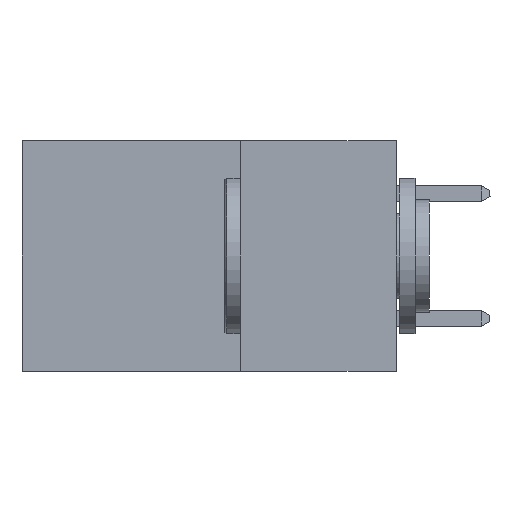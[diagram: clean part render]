
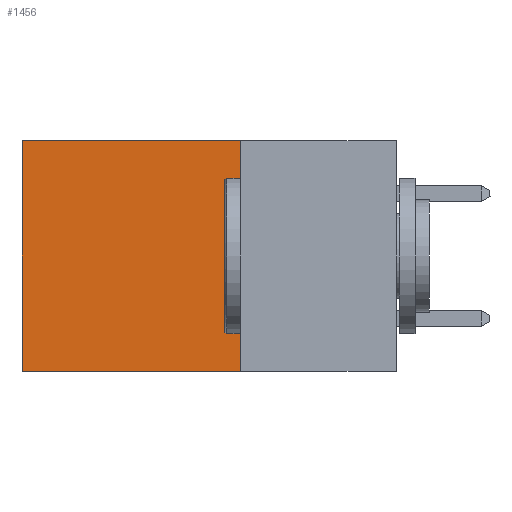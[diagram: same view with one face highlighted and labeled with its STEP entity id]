
A CAD part, left-side view. The second image highlights one B-rep face of the part: STEP entity #1456.
In plain terms, the highlighted planar face has unit normal (-1, 0, 0).
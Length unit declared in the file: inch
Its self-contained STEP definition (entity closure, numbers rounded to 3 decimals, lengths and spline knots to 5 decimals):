
#746 = LINE ( 'NONE', #5062, #2712 ) ;
#984 = VERTEX_POINT ( 'NONE', #23093 ) ;
#1456 = ADVANCED_FACE ( 'NONE', ( #5868 ), #20623, .F. ) ;
#1701 = ORIENTED_EDGE ( 'NONE', *, *, #24674, .T. ) ;
#1760 = VECTOR ( 'NONE', #31688, 39.37008 ) ;
#1788 = DIRECTION ( 'NONE',  ( 0., 1., 0. ) ) ;
#1987 = ORIENTED_EDGE ( 'NONE', *, *, #8417, .F. ) ;
#2712 = VECTOR ( 'NONE', #17250, 39.37008 ) ;
#3353 = LINE ( 'NONE', #26395, #1760 ) ;
#4604 = EDGE_LOOP ( 'NONE', ( #29391, #16786, #1987, #1701 ) ) ;
#5062 = CARTESIAN_POINT ( 'NONE',  ( 0.298, 0.25, -0.37 ) ) ;
#5517 = DIRECTION ( 'NONE',  ( 0., 0., -1. ) ) ;
#5868 = FACE_OUTER_BOUND ( 'NONE', #4604, .T. ) ;
#7280 = EDGE_CURVE ( 'NONE', #13298, #9514, #746, .T. ) ;
#8139 = VERTEX_POINT ( 'NONE', #17391 ) ;
#8417 = EDGE_CURVE ( 'NONE', #8139, #13298, #14065, .T. ) ;
#9514 = VERTEX_POINT ( 'NONE', #31821 ) ;
#9666 = DIRECTION ( 'NONE',  ( 0., 0., -1. ) ) ;
#13298 = VERTEX_POINT ( 'NONE', #14945 ) ;
#14065 = LINE ( 'NONE', #29953, #25134 ) ;
#14945 = CARTESIAN_POINT ( 'NONE',  ( 0.298, 0.25, -0.37 ) ) ;
#15880 = LINE ( 'NONE', #29448, #20218 ) ;
#16786 = ORIENTED_EDGE ( 'NONE', *, *, #7280, .F. ) ;
#17250 = DIRECTION ( 'NONE',  ( 0., 1., 0. ) ) ;
#17391 = CARTESIAN_POINT ( 'NONE',  ( 0.298, 0.25, 0. ) ) ;
#18501 = AXIS2_PLACEMENT_3D ( 'NONE', #30664, #28122, #5517 ) ;
#20218 = VECTOR ( 'NONE', #1788, 39.37008 ) ;
#20623 = PLANE ( 'NONE',  #18501 ) ;
#23093 = CARTESIAN_POINT ( 'NONE',  ( 0.298, 0.6, 0. ) ) ;
#24674 = EDGE_CURVE ( 'NONE', #8139, #984, #15880, .T. ) ;
#25134 = VECTOR ( 'NONE', #9666, 39.37008 ) ;
#26395 = CARTESIAN_POINT ( 'NONE',  ( 0.298, 0.6, 0. ) ) ;
#28122 = DIRECTION ( 'NONE',  ( 1., 0., 0. ) ) ;
#29391 = ORIENTED_EDGE ( 'NONE', *, *, #31599, .T. ) ;
#29448 = CARTESIAN_POINT ( 'NONE',  ( 0.298, 0.25, 0. ) ) ;
#29953 = CARTESIAN_POINT ( 'NONE',  ( 0.298, 0.25, 0. ) ) ;
#30664 = CARTESIAN_POINT ( 'NONE',  ( 0.298, 0.25, 0. ) ) ;
#31599 = EDGE_CURVE ( 'NONE', #984, #9514, #3353, .T. ) ;
#31688 = DIRECTION ( 'NONE',  ( 0., 0., -1. ) ) ;
#31821 = CARTESIAN_POINT ( 'NONE',  ( 0.298, 0.6, -0.37 ) ) ;
